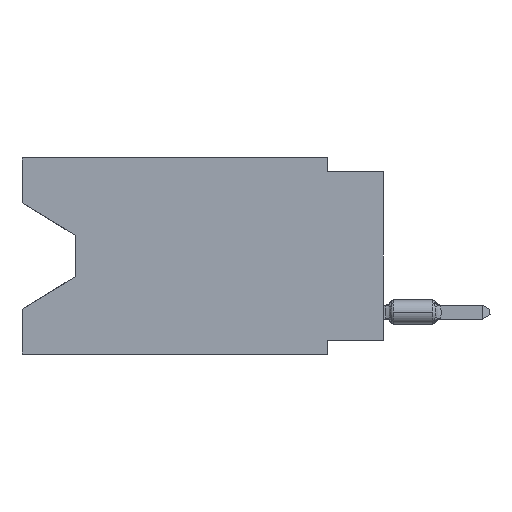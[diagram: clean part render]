
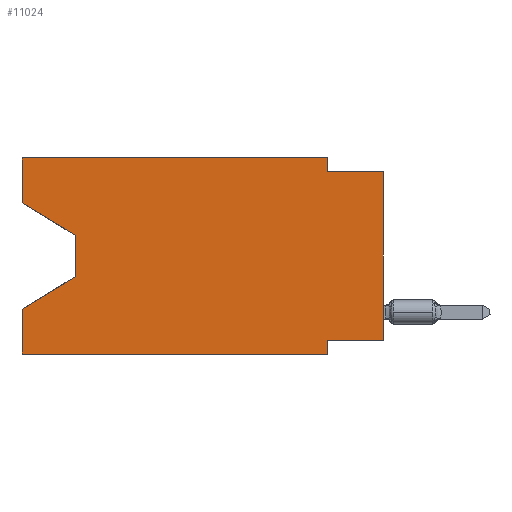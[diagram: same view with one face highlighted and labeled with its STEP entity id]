
A CAD part, left-side view. The second image highlights one B-rep face of the part: STEP entity #11024.
In plain terms, the highlighted planar face has unit normal (-1, 0, 0).
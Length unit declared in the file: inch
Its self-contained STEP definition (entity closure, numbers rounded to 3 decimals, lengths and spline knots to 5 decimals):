
#668 = VECTOR ( 'NONE', #30961, 39.37008 ) ;
#1953 = CARTESIAN_POINT ( 'NONE',  ( 0., 0.645, -0.35 ) ) ;
#2282 = CARTESIAN_POINT ( 'NONE',  ( 0., 0.645, 0. ) ) ;
#2726 = LINE ( 'NONE', #18636, #9509 ) ;
#2892 = VECTOR ( 'NONE', #10838, 39.37008 ) ;
#3619 = EDGE_CURVE ( 'NONE', #9001, #19207, #29047, .T. ) ;
#4144 = VERTEX_POINT ( 'NONE', #21697 ) ;
#4187 = CARTESIAN_POINT ( 'NONE',  ( 0., 0.1, -0.325 ) ) ;
#4959 = LINE ( 'NONE', #1953, #32777 ) ;
#5676 = ORIENTED_EDGE ( 'NONE', *, *, #12140, .F. ) ;
#5981 = EDGE_CURVE ( 'NONE', #33990, #15343, #13963, .T. ) ;
#6370 = DIRECTION ( 'NONE',  ( 0., -0.855, -0.519 ) ) ;
#7012 = CARTESIAN_POINT ( 'NONE',  ( 0., 0.1, -0.35 ) ) ;
#7795 = CARTESIAN_POINT ( 'NONE',  ( 0., 0.55, -0.212 ) ) ;
#8972 = VECTOR ( 'NONE', #6370, 39.37008 ) ;
#9001 = VERTEX_POINT ( 'NONE', #4187 ) ;
#9098 = DIRECTION ( 'NONE',  ( 0., 0., 1. ) ) ;
#9509 = VECTOR ( 'NONE', #36570, 39.37008 ) ;
#9603 = EDGE_CURVE ( 'NONE', #37336, #14835, #11000, .T. ) ;
#9926 = LINE ( 'NONE', #31869, #18347 ) ;
#10831 = ORIENTED_EDGE ( 'NONE', *, *, #16532, .F. ) ;
#10838 = DIRECTION ( 'NONE',  ( 0., 0.855, -0.519 ) ) ;
#10964 = EDGE_LOOP ( 'NONE', ( #22858, #37044, #28779, #17016, #38414, #23677, #13055, #11448, #5676, #20944, #10831, #20824 ) ) ;
#11000 = LINE ( 'NONE', #35539, #22929 ) ;
#11024 = ADVANCED_FACE ( 'NONE', ( #25503 ), #31737, .F. ) ;
#11395 = CARTESIAN_POINT ( 'NONE',  ( 0., 0., -0.025 ) ) ;
#11397 = DIRECTION ( 'NONE',  ( 0., 0., -1. ) ) ;
#11448 = ORIENTED_EDGE ( 'NONE', *, *, #18104, .T. ) ;
#11867 = DIRECTION ( 'NONE',  ( 0., 1., 0. ) ) ;
#12051 = CARTESIAN_POINT ( 'NONE',  ( 0., 0.1, 0. ) ) ;
#12140 = EDGE_CURVE ( 'NONE', #14835, #25831, #37391, .T. ) ;
#12753 = CARTESIAN_POINT ( 'NONE',  ( 0., 0.645, -0.35 ) ) ;
#12826 = CARTESIAN_POINT ( 'NONE',  ( 0., 0.645, -0.08025 ) ) ;
#12932 = VERTEX_POINT ( 'NONE', #12753 ) ;
#13023 = VERTEX_POINT ( 'NONE', #22402 ) ;
#13026 = CARTESIAN_POINT ( 'NONE',  ( 0., 0.645, 0. ) ) ;
#13055 = ORIENTED_EDGE ( 'NONE', *, *, #21215, .F. ) ;
#13556 = EDGE_CURVE ( 'NONE', #12932, #19207, #4959, .T. ) ;
#13564 = CARTESIAN_POINT ( 'NONE',  ( 0., 0.1, -0.35 ) ) ;
#13963 = LINE ( 'NONE', #29846, #33691 ) ;
#14835 = VERTEX_POINT ( 'NONE', #31108 ) ;
#15343 = VERTEX_POINT ( 'NONE', #15763 ) ;
#15763 = CARTESIAN_POINT ( 'NONE',  ( 0., 0.55, -0.212 ) ) ;
#15790 = EDGE_CURVE ( 'NONE', #15343, #13023, #17434, .T. ) ;
#16435 = DIRECTION ( 'NONE',  ( 1., 0., 0. ) ) ;
#16532 = EDGE_CURVE ( 'NONE', #24302, #37336, #9926, .T. ) ;
#17016 = ORIENTED_EDGE ( 'NONE', *, *, #27899, .F. ) ;
#17434 = LINE ( 'NONE', #7795, #2892 ) ;
#17686 = VECTOR ( 'NONE', #9098, 39.37008 ) ;
#17900 = CARTESIAN_POINT ( 'NONE',  ( 0., 0., -0.325 ) ) ;
#18013 = CARTESIAN_POINT ( 'NONE',  ( 0., 0., -0.325 ) ) ;
#18104 = EDGE_CURVE ( 'NONE', #34808, #25831, #33261, .T. ) ;
#18347 = VECTOR ( 'NONE', #18776, 39.37008 ) ;
#18497 = VECTOR ( 'NONE', #35299, 39.37008 ) ;
#18636 = CARTESIAN_POINT ( 'NONE',  ( 0., 0.645, 0. ) ) ;
#18776 = DIRECTION ( 'NONE',  ( 0., -1., 0. ) ) ;
#19077 = AXIS2_PLACEMENT_3D ( 'NONE', #13026, #16435, #34577 ) ;
#19207 = VERTEX_POINT ( 'NONE', #7012 ) ;
#20401 = DIRECTION ( 'NONE',  ( 0., 0., -1. ) ) ;
#20477 = CARTESIAN_POINT ( 'NONE',  ( 0., 0.645, 0. ) ) ;
#20824 = ORIENTED_EDGE ( 'NONE', *, *, #36349, .F. ) ;
#20944 = ORIENTED_EDGE ( 'NONE', *, *, #9603, .F. ) ;
#21215 = EDGE_CURVE ( 'NONE', #34808, #9001, #36637, .T. ) ;
#21697 = CARTESIAN_POINT ( 'NONE',  ( 0., 0.645, -0.08025 ) ) ;
#21880 = LINE ( 'NONE', #12826, #8972 ) ;
#22402 = CARTESIAN_POINT ( 'NONE',  ( 0., 0.645, -0.26975 ) ) ;
#22858 = ORIENTED_EDGE ( 'NONE', *, *, #24338, .T. ) ;
#22929 = VECTOR ( 'NONE', #11397, 39.37008 ) ;
#23677 = ORIENTED_EDGE ( 'NONE', *, *, #3619, .F. ) ;
#24187 = CARTESIAN_POINT ( 'NONE',  ( 0., 0., 0. ) ) ;
#24302 = VERTEX_POINT ( 'NONE', #20477 ) ;
#24338 = EDGE_CURVE ( 'NONE', #4144, #33990, #21880, .T. ) ;
#24421 = LINE ( 'NONE', #2282, #35862 ) ;
#24961 = VECTOR ( 'NONE', #11867, 39.37008 ) ;
#25503 = FACE_OUTER_BOUND ( 'NONE', #10964, .T. ) ;
#25831 = VERTEX_POINT ( 'NONE', #11395 ) ;
#26494 = DIRECTION ( 'NONE',  ( 0., -1., 0. ) ) ;
#26838 = CARTESIAN_POINT ( 'NONE',  ( 0., 0.55, -0.138 ) ) ;
#27899 = EDGE_CURVE ( 'NONE', #12932, #13023, #2726, .T. ) ;
#28779 = ORIENTED_EDGE ( 'NONE', *, *, #15790, .T. ) ;
#29047 = LINE ( 'NONE', #13564, #18497 ) ;
#29846 = CARTESIAN_POINT ( 'NONE',  ( 0., 0.55, -0.138 ) ) ;
#30768 = CARTESIAN_POINT ( 'NONE',  ( 0., 0., -0.025 ) ) ;
#30961 = DIRECTION ( 'NONE',  ( 0., -1., 0. ) ) ;
#31108 = CARTESIAN_POINT ( 'NONE',  ( 0., 0.1, -0.025 ) ) ;
#31737 = PLANE ( 'NONE',  #19077 ) ;
#31869 = CARTESIAN_POINT ( 'NONE',  ( 0., 0.645, 0. ) ) ;
#32777 = VECTOR ( 'NONE', #26494, 39.37008 ) ;
#33261 = LINE ( 'NONE', #24187, #17686 ) ;
#33672 = DIRECTION ( 'NONE',  ( 0., 0., 1. ) ) ;
#33691 = VECTOR ( 'NONE', #20401, 39.37008 ) ;
#33990 = VERTEX_POINT ( 'NONE', #26838 ) ;
#34577 = DIRECTION ( 'NONE',  ( 0., 0., -1. ) ) ;
#34808 = VERTEX_POINT ( 'NONE', #18013 ) ;
#35299 = DIRECTION ( 'NONE',  ( 0., 0., -1. ) ) ;
#35539 = CARTESIAN_POINT ( 'NONE',  ( 0., 0.1, 0. ) ) ;
#35862 = VECTOR ( 'NONE', #33672, 39.37008 ) ;
#36349 = EDGE_CURVE ( 'NONE', #4144, #24302, #24421, .T. ) ;
#36570 = DIRECTION ( 'NONE',  ( 0., 0., 1. ) ) ;
#36637 = LINE ( 'NONE', #17900, #24961 ) ;
#37044 = ORIENTED_EDGE ( 'NONE', *, *, #5981, .T. ) ;
#37336 = VERTEX_POINT ( 'NONE', #12051 ) ;
#37391 = LINE ( 'NONE', #30768, #668 ) ;
#38414 = ORIENTED_EDGE ( 'NONE', *, *, #13556, .T. ) ;
